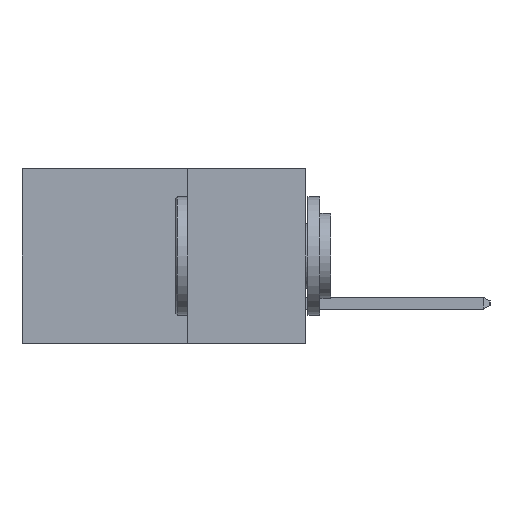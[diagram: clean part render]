
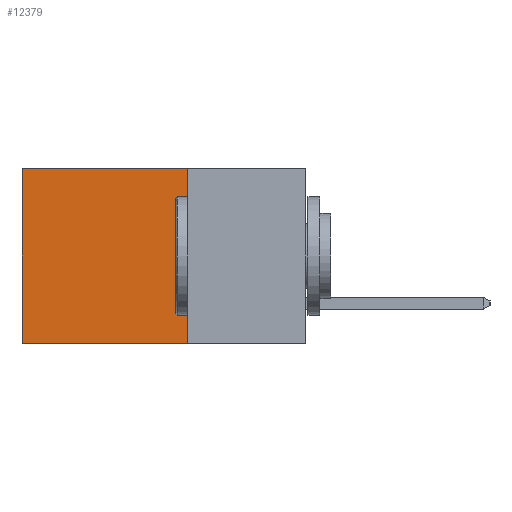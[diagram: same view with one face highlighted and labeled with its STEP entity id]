
A CAD part, left-side view. The second image highlights one B-rep face of the part: STEP entity #12379.
In plain terms, the highlighted planar face has unit normal (-1, 0, 0).
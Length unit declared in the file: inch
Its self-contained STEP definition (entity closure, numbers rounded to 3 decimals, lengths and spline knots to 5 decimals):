
#363 = VERTEX_POINT ( 'NONE', #6426 ) ;
#564 = VECTOR ( 'NONE', #15074, 39.37008 ) ;
#925 = VECTOR ( 'NONE', #3202, 39.37008 ) ;
#1343 = LINE ( 'NONE', #11800, #925 ) ;
#1454 = EDGE_CURVE ( 'NONE', #11521, #6719, #1343, .T. ) ;
#1632 = ORIENTED_EDGE ( 'NONE', *, *, #5204, .T. ) ;
#1723 = DIRECTION ( 'NONE',  ( 0., 0., -1. ) ) ;
#2299 = LINE ( 'NONE', #10160, #14514 ) ;
#2964 = EDGE_LOOP ( 'NONE', ( #12062, #14820, #8637, #1632 ) ) ;
#3085 = PLANE ( 'NONE',  #7435 ) ;
#3102 = VERTEX_POINT ( 'NONE', #7735 ) ;
#3202 = DIRECTION ( 'NONE',  ( 0., 0., -1. ) ) ;
#3667 = VECTOR ( 'NONE', #9350, 39.37008 ) ;
#4220 = LINE ( 'NONE', #4240, #564 ) ;
#4240 = CARTESIAN_POINT ( 'NONE',  ( 0.298, 0.25, 0. ) ) ;
#4284 = DIRECTION ( 'NONE',  ( 1., 0., 0. ) ) ;
#5204 = EDGE_CURVE ( 'NONE', #3102, #11521, #4220, .T. ) ;
#5933 = EDGE_CURVE ( 'NONE', #363, #6719, #7203, .T. ) ;
#6426 = CARTESIAN_POINT ( 'NONE',  ( 0.298, 0.25, -0.37 ) ) ;
#6719 = VERTEX_POINT ( 'NONE', #8784 ) ;
#7203 = LINE ( 'NONE', #9281, #3667 ) ;
#7435 = AXIS2_PLACEMENT_3D ( 'NONE', #11620, #4284, #12916 ) ;
#7735 = CARTESIAN_POINT ( 'NONE',  ( 0.298, 0.25, 0. ) ) ;
#8637 = ORIENTED_EDGE ( 'NONE', *, *, #9897, .F. ) ;
#8647 = CARTESIAN_POINT ( 'NONE',  ( 0.298, 0.6, 0. ) ) ;
#8784 = CARTESIAN_POINT ( 'NONE',  ( 0.298, 0.6, -0.37 ) ) ;
#9281 = CARTESIAN_POINT ( 'NONE',  ( 0.298, 0.25, -0.37 ) ) ;
#9350 = DIRECTION ( 'NONE',  ( 0., 1., 0. ) ) ;
#9897 = EDGE_CURVE ( 'NONE', #3102, #363, #2299, .T. ) ;
#10160 = CARTESIAN_POINT ( 'NONE',  ( 0.298, 0.25, 0. ) ) ;
#11521 = VERTEX_POINT ( 'NONE', #8647 ) ;
#11620 = CARTESIAN_POINT ( 'NONE',  ( 0.298, 0.25, 0. ) ) ;
#11800 = CARTESIAN_POINT ( 'NONE',  ( 0.298, 0.6, 0. ) ) ;
#12062 = ORIENTED_EDGE ( 'NONE', *, *, #1454, .T. ) ;
#12379 = ADVANCED_FACE ( 'NONE', ( #15752 ), #3085, .F. ) ;
#12916 = DIRECTION ( 'NONE',  ( 0., 0., -1. ) ) ;
#14514 = VECTOR ( 'NONE', #1723, 39.37008 ) ;
#14820 = ORIENTED_EDGE ( 'NONE', *, *, #5933, .F. ) ;
#15074 = DIRECTION ( 'NONE',  ( 0., 1., 0. ) ) ;
#15752 = FACE_OUTER_BOUND ( 'NONE', #2964, .T. ) ;
